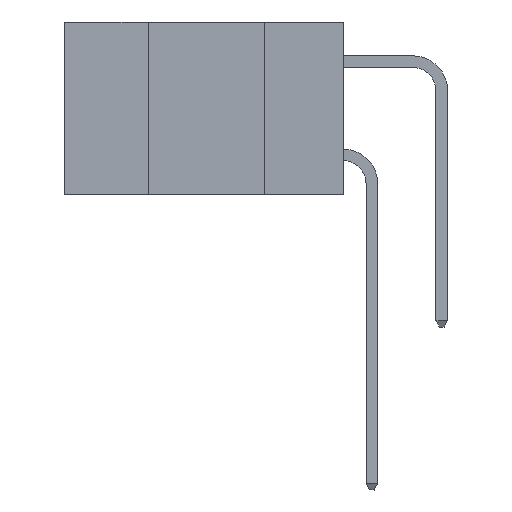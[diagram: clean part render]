
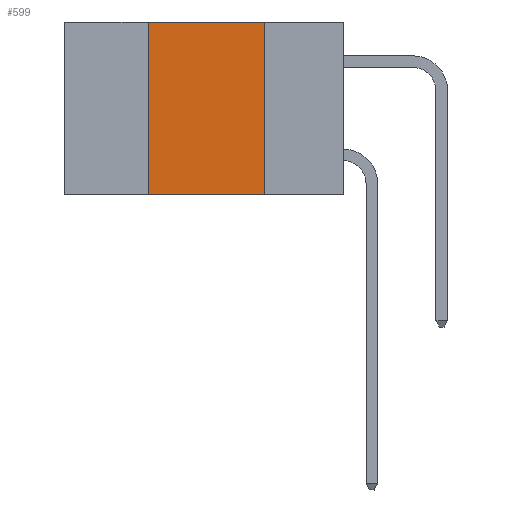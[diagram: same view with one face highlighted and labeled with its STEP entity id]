
A CAD part, left-side view. The second image highlights one B-rep face of the part: STEP entity #599.
In plain terms, the highlighted planar face has unit normal (-1, 0, 0).
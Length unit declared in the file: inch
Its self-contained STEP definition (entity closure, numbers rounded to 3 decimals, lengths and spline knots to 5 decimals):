
#166 = CARTESIAN_POINT ( 'NONE',  ( 0., 0.17, -0.37 ) ) ;
#241 = CARTESIAN_POINT ( 'NONE',  ( 0., 0.6, 0. ) ) ;
#377 = DIRECTION ( 'NONE',  ( 0., -1., 0. ) ) ;
#450 = LINE ( 'NONE', #13345, #10644 ) ;
#599 = ADVANCED_FACE ( 'NONE', ( #14688 ), #1733, .F. ) ;
#1337 = EDGE_CURVE ( 'NONE', #14206, #2451, #11937, .T. ) ;
#1408 = EDGE_CURVE ( 'NONE', #2451, #14108, #9478, .T. ) ;
#1733 = PLANE ( 'NONE',  #8887 ) ;
#2451 = VERTEX_POINT ( 'NONE', #3451 ) ;
#2992 = EDGE_CURVE ( 'NONE', #8749, #14206, #8824, .T. ) ;
#3092 = DIRECTION ( 'NONE',  ( 0., 0., -1. ) ) ;
#3451 = CARTESIAN_POINT ( 'NONE',  ( 0., 0.17, 0. ) ) ;
#5185 = CARTESIAN_POINT ( 'NONE',  ( 0., 0.17, -0.37 ) ) ;
#5277 = EDGE_LOOP ( 'NONE', ( #14676, #8176, #11459, #8246 ) ) ;
#5524 = CARTESIAN_POINT ( 'NONE',  ( 0., 0.6, 0. ) ) ;
#8176 = ORIENTED_EDGE ( 'NONE', *, *, #1337, .F. ) ;
#8246 = ORIENTED_EDGE ( 'NONE', *, *, #10663, .T. ) ;
#8473 = VECTOR ( 'NONE', #12850, 39.37008 ) ;
#8749 = VERTEX_POINT ( 'NONE', #11313 ) ;
#8824 = LINE ( 'NONE', #11285, #13141 ) ;
#8887 = AXIS2_PLACEMENT_3D ( 'NONE', #5524, #12333, #3092 ) ;
#9478 = LINE ( 'NONE', #166, #8473 ) ;
#10644 = VECTOR ( 'NONE', #377, 39.37008 ) ;
#10663 = EDGE_CURVE ( 'NONE', #8749, #14108, #450, .T. ) ;
#10790 = DIRECTION ( 'NONE',  ( 0., -1., 0. ) ) ;
#11231 = CARTESIAN_POINT ( 'NONE',  ( 0., 0.42, 0. ) ) ;
#11285 = CARTESIAN_POINT ( 'NONE',  ( 0., 0.42, -0.37 ) ) ;
#11313 = CARTESIAN_POINT ( 'NONE',  ( 0., 0.42, -0.37 ) ) ;
#11459 = ORIENTED_EDGE ( 'NONE', *, *, #2992, .F. ) ;
#11937 = LINE ( 'NONE', #241, #14061 ) ;
#12333 = DIRECTION ( 'NONE',  ( 1., 0., 0. ) ) ;
#12850 = DIRECTION ( 'NONE',  ( 0., 0., -1. ) ) ;
#13141 = VECTOR ( 'NONE', #13489, 39.37008 ) ;
#13345 = CARTESIAN_POINT ( 'NONE',  ( 0., 0.6, -0.37 ) ) ;
#13489 = DIRECTION ( 'NONE',  ( 0., 0., 1. ) ) ;
#14061 = VECTOR ( 'NONE', #10790, 39.37008 ) ;
#14108 = VERTEX_POINT ( 'NONE', #5185 ) ;
#14206 = VERTEX_POINT ( 'NONE', #11231 ) ;
#14676 = ORIENTED_EDGE ( 'NONE', *, *, #1408, .F. ) ;
#14688 = FACE_OUTER_BOUND ( 'NONE', #5277, .T. ) ;
